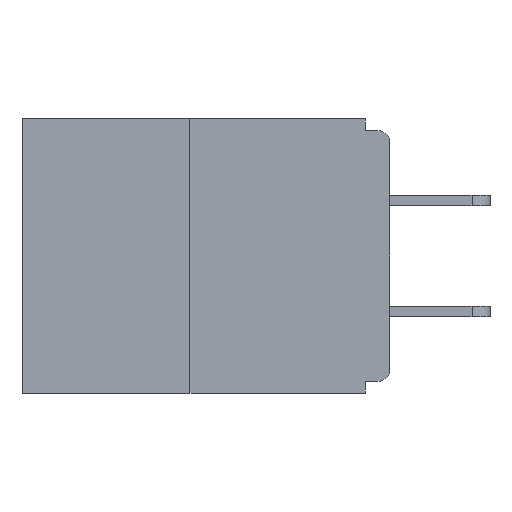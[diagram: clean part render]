
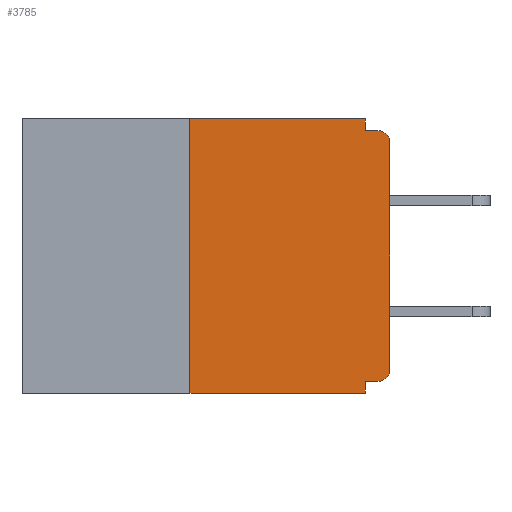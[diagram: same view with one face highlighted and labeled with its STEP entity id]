
A CAD part, left-side view. The second image highlights one B-rep face of the part: STEP entity #3785.
In plain terms, the highlighted planar face has unit normal (-1, 0, 0).
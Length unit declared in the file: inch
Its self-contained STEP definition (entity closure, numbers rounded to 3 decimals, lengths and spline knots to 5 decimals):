
#12 = DIRECTION ( 'NONE',  ( 0., 0., -1. ) ) ;
#406 = CARTESIAN_POINT ( 'NONE',  ( 0., 0.46, 0. ) ) ;
#608 = LINE ( 'NONE', #7180, #10396 ) ;
#1157 = ORIENTED_EDGE ( 'NONE', *, *, #5184, .T. ) ;
#1280 = CARTESIAN_POINT ( 'NONE',  ( 0., 0., -0.03 ) ) ;
#1362 = ORIENTED_EDGE ( 'NONE', *, *, #1883, .F. ) ;
#1501 = ORIENTED_EDGE ( 'NONE', *, *, #21229, .F. ) ;
#1648 = CARTESIAN_POINT ( 'NONE',  ( 0., 0.25, 0. ) ) ;
#1783 = EDGE_CURVE ( 'NONE', #8008, #24992, #18072, .T. ) ;
#1883 = EDGE_CURVE ( 'NONE', #8008, #6696, #608, .T. ) ;
#1980 = DIRECTION ( 'NONE',  ( 0., 0., 1. ) ) ;
#1981 = DIRECTION ( 'NONE',  ( -1., 0., 0. ) ) ;
#2310 = DIRECTION ( 'NONE',  ( 0., 0., -1. ) ) ;
#2376 = DIRECTION ( 'NONE',  ( 0., -1., 0. ) ) ;
#2406 = ORIENTED_EDGE ( 'NONE', *, *, #6602, .T. ) ;
#3135 = ORIENTED_EDGE ( 'NONE', *, *, #9156, .T. ) ;
#3193 = CARTESIAN_POINT ( 'NONE',  ( 0., 0.25, -0.343 ) ) ;
#3690 = DIRECTION ( 'NONE',  ( 0., 0., -1. ) ) ;
#3770 = DIRECTION ( 'NONE',  ( 0., 0., 1. ) ) ;
#3785 = ADVANCED_FACE ( 'NONE', ( #24608 ), #9647, .F. ) ;
#3960 = AXIS2_PLACEMENT_3D ( 'NONE', #9566, #1981, #11615 ) ;
#4027 = DIRECTION ( 'NONE',  ( -1., 0., 0. ) ) ;
#4472 = CARTESIAN_POINT ( 'NONE',  ( 0., 0.031, -0.328 ) ) ;
#4593 = LINE ( 'NONE', #18379, #21161 ) ;
#5184 = EDGE_CURVE ( 'NONE', #23382, #19174, #6408, .T. ) ;
#5262 = ORIENTED_EDGE ( 'NONE', *, *, #22878, .F. ) ;
#5460 = CARTESIAN_POINT ( 'NONE',  ( 0., 0.031, -0.343 ) ) ;
#5516 = VERTEX_POINT ( 'NONE', #15381 ) ;
#6355 = ORIENTED_EDGE ( 'NONE', *, *, #15943, .F. ) ;
#6408 = CIRCLE ( 'NONE', #24257, 0.015 ) ;
#6602 = EDGE_CURVE ( 'NONE', #19174, #15045, #22562, .T. ) ;
#6658 = DIRECTION ( 'NONE',  ( 0., 0., -1. ) ) ;
#6696 = VERTEX_POINT ( 'NONE', #1648 ) ;
#6909 = VERTEX_POINT ( 'NONE', #24179 ) ;
#7180 = CARTESIAN_POINT ( 'NONE',  ( 0., 0.25, 0. ) ) ;
#7655 = CARTESIAN_POINT ( 'NONE',  ( 0., 0., -0.313 ) ) ;
#8008 = VERTEX_POINT ( 'NONE', #3193 ) ;
#8160 = CARTESIAN_POINT ( 'NONE',  ( 0., 0., -0.015 ) ) ;
#8318 = VERTEX_POINT ( 'NONE', #4472 ) ;
#8583 = CARTESIAN_POINT ( 'NONE',  ( 0., 0.031, 0. ) ) ;
#9156 = EDGE_CURVE ( 'NONE', #15045, #5516, #19985, .T. ) ;
#9353 = LINE ( 'NONE', #15952, #17945 ) ;
#9418 = CARTESIAN_POINT ( 'NONE',  ( 0., 0., 0. ) ) ;
#9566 = CARTESIAN_POINT ( 'NONE',  ( 0., 0.015, -0.03 ) ) ;
#9647 = PLANE ( 'NONE',  #17260 ) ;
#10022 = LINE ( 'NONE', #17391, #10916 ) ;
#10023 = EDGE_LOOP ( 'NONE', ( #16949, #1362, #23873, #1501, #5262, #1157, #2406, #3135, #6355, #22633 ) ) ;
#10190 = DIRECTION ( 'NONE',  ( 0., 1., 0. ) ) ;
#10396 = VECTOR ( 'NONE', #1980, 39.37008 ) ;
#10916 = VECTOR ( 'NONE', #12, 39.37008 ) ;
#10979 = VECTOR ( 'NONE', #23887, 39.37008 ) ;
#11615 = DIRECTION ( 'NONE',  ( 0., 0., -1. ) ) ;
#11703 = EDGE_CURVE ( 'NONE', #6696, #12555, #9353, .T. ) ;
#12196 = DIRECTION ( 'NONE',  ( 1., 0., 0. ) ) ;
#12396 = LINE ( 'NONE', #16026, #16702 ) ;
#12555 = VERTEX_POINT ( 'NONE', #8583 ) ;
#12803 = DIRECTION ( 'NONE',  ( 0., -1., 0. ) ) ;
#12879 = CARTESIAN_POINT ( 'NONE',  ( 0., 0.46, -0.343 ) ) ;
#14381 = CARTESIAN_POINT ( 'NONE',  ( 0., 0.015, -0.328 ) ) ;
#15045 = VERTEX_POINT ( 'NONE', #1280 ) ;
#15381 = CARTESIAN_POINT ( 'NONE',  ( 0., 0.015, -0.015 ) ) ;
#15599 = CARTESIAN_POINT ( 'NONE',  ( 0., 0.015, -0.313 ) ) ;
#15901 = LINE ( 'NONE', #8160, #10979 ) ;
#15943 = EDGE_CURVE ( 'NONE', #6909, #5516, #15901, .T. ) ;
#15952 = CARTESIAN_POINT ( 'NONE',  ( 0., 0.46, 0. ) ) ;
#16026 = CARTESIAN_POINT ( 'NONE',  ( 0., 0., -0.328 ) ) ;
#16531 = EDGE_CURVE ( 'NONE', #12555, #6909, #10022, .T. ) ;
#16702 = VECTOR ( 'NONE', #10190, 39.37008 ) ;
#16827 = VECTOR ( 'NONE', #12803, 39.37008 ) ;
#16949 = ORIENTED_EDGE ( 'NONE', *, *, #11703, .F. ) ;
#17260 = AXIS2_PLACEMENT_3D ( 'NONE', #406, #12196, #2310 ) ;
#17391 = CARTESIAN_POINT ( 'NONE',  ( 0., 0.031, 0. ) ) ;
#17945 = VECTOR ( 'NONE', #2376, 39.37008 ) ;
#18072 = LINE ( 'NONE', #12879, #16827 ) ;
#18379 = CARTESIAN_POINT ( 'NONE',  ( 0., 0.031, -0.343 ) ) ;
#19174 = VERTEX_POINT ( 'NONE', #7655 ) ;
#19985 = CIRCLE ( 'NONE', #3960, 0.015 ) ;
#21161 = VECTOR ( 'NONE', #6658, 39.37008 ) ;
#21229 = EDGE_CURVE ( 'NONE', #8318, #24992, #4593, .T. ) ;
#21958 = VECTOR ( 'NONE', #3770, 39.37008 ) ;
#22562 = LINE ( 'NONE', #9418, #21958 ) ;
#22633 = ORIENTED_EDGE ( 'NONE', *, *, #16531, .F. ) ;
#22878 = EDGE_CURVE ( 'NONE', #23382, #8318, #12396, .T. ) ;
#23382 = VERTEX_POINT ( 'NONE', #14381 ) ;
#23873 = ORIENTED_EDGE ( 'NONE', *, *, #1783, .T. ) ;
#23887 = DIRECTION ( 'NONE',  ( 0., -1., 0. ) ) ;
#24179 = CARTESIAN_POINT ( 'NONE',  ( 0., 0.031, -0.015 ) ) ;
#24257 = AXIS2_PLACEMENT_3D ( 'NONE', #15599, #4027, #3690 ) ;
#24608 = FACE_OUTER_BOUND ( 'NONE', #10023, .T. ) ;
#24992 = VERTEX_POINT ( 'NONE', #5460 ) ;
